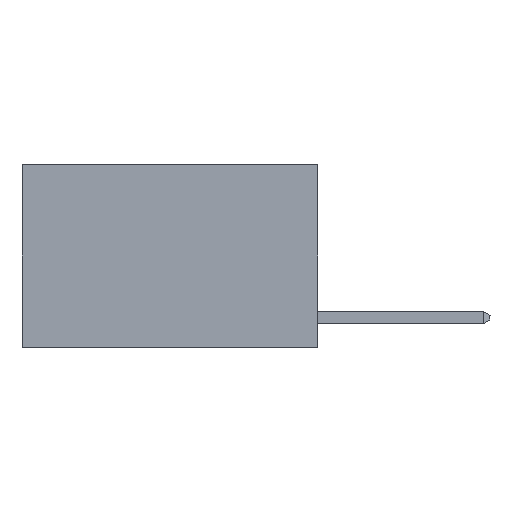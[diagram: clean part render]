
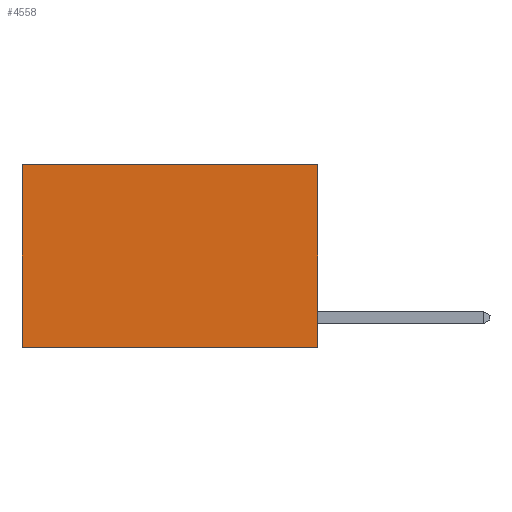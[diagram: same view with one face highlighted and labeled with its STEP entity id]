
A CAD part, left-side view. The second image highlights one B-rep face of the part: STEP entity #4558.
In plain terms, the highlighted planar face has unit normal (-1, 0, 0).
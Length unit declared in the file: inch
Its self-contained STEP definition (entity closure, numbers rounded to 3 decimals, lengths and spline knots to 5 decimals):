
#379 = CARTESIAN_POINT ( 'NONE',  ( 0.2625, 0.6, 0. ) ) ;
#957 = DIRECTION ( 'NONE',  ( 0., 1., 0. ) ) ;
#1689 = CARTESIAN_POINT ( 'NONE',  ( 0.2625, 0.6, -0.37 ) ) ;
#2166 = CARTESIAN_POINT ( 'NONE',  ( 0.2625, 0., 0. ) ) ;
#2638 = LINE ( 'NONE', #10759, #9327 ) ;
#2981 = VERTEX_POINT ( 'NONE', #10089 ) ;
#3091 = LINE ( 'NONE', #15220, #10245 ) ;
#3119 = EDGE_CURVE ( 'NONE', #2981, #9765, #15312, .T. ) ;
#3384 = EDGE_LOOP ( 'NONE', ( #15978, #11395, #9582, #17366 ) ) ;
#4558 = ADVANCED_FACE ( 'NONE', ( #13626 ), #5063, .F. ) ;
#5063 = PLANE ( 'NONE',  #16850 ) ;
#6486 = DIRECTION ( 'NONE',  ( 0., 0., -1. ) ) ;
#6524 = VERTEX_POINT ( 'NONE', #10459 ) ;
#7703 = VECTOR ( 'NONE', #11802, 39.37008 ) ;
#7947 = CARTESIAN_POINT ( 'NONE',  ( 0.2625, 0., 0. ) ) ;
#8086 = EDGE_CURVE ( 'NONE', #10881, #6524, #13735, .T. ) ;
#8189 = CARTESIAN_POINT ( 'NONE',  ( 0.2625, 0., 0. ) ) ;
#9327 = VECTOR ( 'NONE', #9328, 39.37008 ) ;
#9328 = DIRECTION ( 'NONE',  ( 0., 1., 0. ) ) ;
#9368 = DIRECTION ( 'NONE',  ( 0., 0., -1. ) ) ;
#9582 = ORIENTED_EDGE ( 'NONE', *, *, #8086, .F. ) ;
#9765 = VERTEX_POINT ( 'NONE', #1689 ) ;
#9938 = VECTOR ( 'NONE', #9368, 39.37008 ) ;
#10089 = CARTESIAN_POINT ( 'NONE',  ( 0.2625, 0.6, 0. ) ) ;
#10245 = VECTOR ( 'NONE', #957, 39.37008 ) ;
#10459 = CARTESIAN_POINT ( 'NONE',  ( 0.2625, 0., -0.37 ) ) ;
#10759 = CARTESIAN_POINT ( 'NONE',  ( 0.2625, 0., 0. ) ) ;
#10881 = VERTEX_POINT ( 'NONE', #8189 ) ;
#11395 = ORIENTED_EDGE ( 'NONE', *, *, #13376, .F. ) ;
#11802 = DIRECTION ( 'NONE',  ( 0., 0., -1. ) ) ;
#13376 = EDGE_CURVE ( 'NONE', #6524, #9765, #3091, .T. ) ;
#13626 = FACE_OUTER_BOUND ( 'NONE', #3384, .T. ) ;
#13735 = LINE ( 'NONE', #7947, #9938 ) ;
#13897 = EDGE_CURVE ( 'NONE', #10881, #2981, #2638, .T. ) ;
#15037 = DIRECTION ( 'NONE',  ( 1., 0., 0. ) ) ;
#15220 = CARTESIAN_POINT ( 'NONE',  ( 0.2625, 0., -0.37 ) ) ;
#15312 = LINE ( 'NONE', #379, #7703 ) ;
#15978 = ORIENTED_EDGE ( 'NONE', *, *, #3119, .T. ) ;
#16850 = AXIS2_PLACEMENT_3D ( 'NONE', #2166, #15037, #6486 ) ;
#17366 = ORIENTED_EDGE ( 'NONE', *, *, #13897, .T. ) ;
